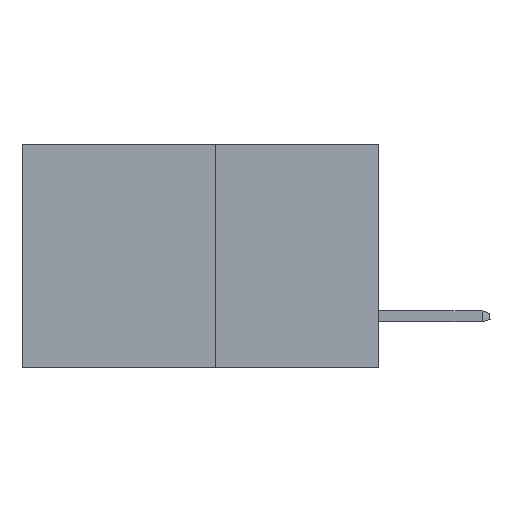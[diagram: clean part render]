
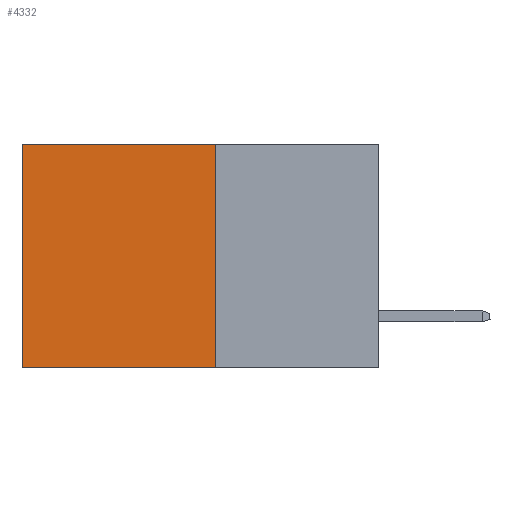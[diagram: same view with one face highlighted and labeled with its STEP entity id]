
A CAD part, left-side view. The second image highlights one B-rep face of the part: STEP entity #4332.
In plain terms, the highlighted planar face has unit normal (-1, 0, 0).
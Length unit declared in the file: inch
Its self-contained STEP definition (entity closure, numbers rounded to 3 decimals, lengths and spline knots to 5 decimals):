
#315 = EDGE_CURVE ( 'NONE', #20662, #1093, #8728, .T. ) ;
#1093 = VERTEX_POINT ( 'NONE', #16530 ) ;
#2475 = LINE ( 'NONE', #7646, #11137 ) ;
#3926 = LINE ( 'NONE', #12534, #17152 ) ;
#4132 = VECTOR ( 'NONE', #8910, 39.37008 ) ;
#4332 = ADVANCED_FACE ( 'NONE', ( #20539 ), #11135, .F. ) ;
#4735 = ORIENTED_EDGE ( 'NONE', *, *, #315, .T. ) ;
#4944 = VERTEX_POINT ( 'NONE', #18491 ) ;
#6372 = ORIENTED_EDGE ( 'NONE', *, *, #19164, .F. ) ;
#7646 = CARTESIAN_POINT ( 'NONE',  ( 0.277, 0.27, 0. ) ) ;
#7881 = AXIS2_PLACEMENT_3D ( 'NONE', #10959, #10438, #10435 ) ;
#8728 = LINE ( 'NONE', #22163, #4132 ) ;
#8910 = DIRECTION ( 'NONE',  ( 0., 0., -1. ) ) ;
#9347 = DIRECTION ( 'NONE',  ( 0., 1., 0. ) ) ;
#9503 = VERTEX_POINT ( 'NONE', #22081 ) ;
#9749 = EDGE_LOOP ( 'NONE', ( #4735, #14971, #6372, #15801 ) ) ;
#10435 = DIRECTION ( 'NONE',  ( 0., 0., -1. ) ) ;
#10438 = DIRECTION ( 'NONE',  ( 1., 0., 0. ) ) ;
#10959 = CARTESIAN_POINT ( 'NONE',  ( 0.277, 0.27, -0.37 ) ) ;
#11135 = PLANE ( 'NONE',  #7881 ) ;
#11137 = VECTOR ( 'NONE', #9347, 39.37008 ) ;
#12534 = CARTESIAN_POINT ( 'NONE',  ( 0.277, 0.27, -0.37 ) ) ;
#14168 = EDGE_CURVE ( 'NONE', #4944, #1093, #3926, .T. ) ;
#14232 = LINE ( 'NONE', #19289, #17753 ) ;
#14274 = DIRECTION ( 'NONE',  ( 0., 1., 0. ) ) ;
#14971 = ORIENTED_EDGE ( 'NONE', *, *, #14168, .F. ) ;
#15801 = ORIENTED_EDGE ( 'NONE', *, *, #21468, .T. ) ;
#16530 = CARTESIAN_POINT ( 'NONE',  ( 0.277, 0.59, -0.37 ) ) ;
#17152 = VECTOR ( 'NONE', #14274, 39.37008 ) ;
#17753 = VECTOR ( 'NONE', #20924, 39.37008 ) ;
#18491 = CARTESIAN_POINT ( 'NONE',  ( 0.277, 0.27, -0.37 ) ) ;
#19164 = EDGE_CURVE ( 'NONE', #9503, #4944, #14232, .T. ) ;
#19289 = CARTESIAN_POINT ( 'NONE',  ( 0.277, 0.27, -0.37 ) ) ;
#19737 = CARTESIAN_POINT ( 'NONE',  ( 0.277, 0.59, 0. ) ) ;
#20539 = FACE_OUTER_BOUND ( 'NONE', #9749, .T. ) ;
#20662 = VERTEX_POINT ( 'NONE', #19737 ) ;
#20924 = DIRECTION ( 'NONE',  ( 0., 0., -1. ) ) ;
#21468 = EDGE_CURVE ( 'NONE', #9503, #20662, #2475, .T. ) ;
#22081 = CARTESIAN_POINT ( 'NONE',  ( 0.277, 0.27, 0. ) ) ;
#22163 = CARTESIAN_POINT ( 'NONE',  ( 0.277, 0.59, -0.37 ) ) ;
